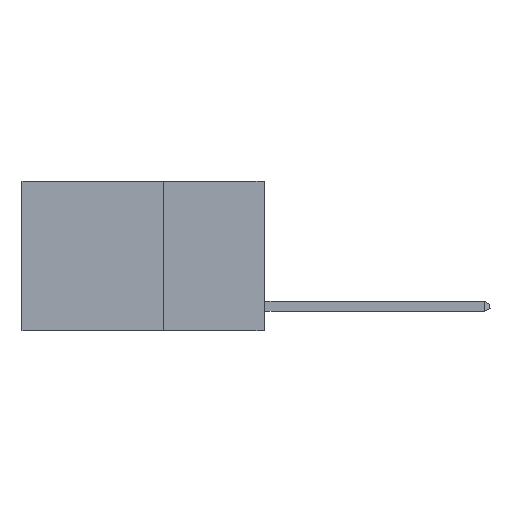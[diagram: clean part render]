
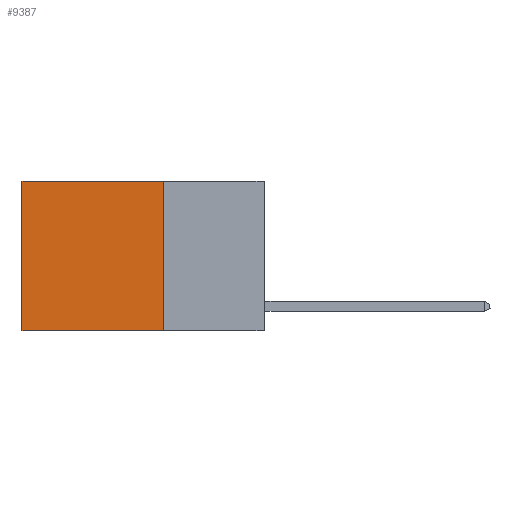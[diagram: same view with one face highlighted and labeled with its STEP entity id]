
A CAD part, left-side view. The second image highlights one B-rep face of the part: STEP entity #9387.
In plain terms, the highlighted planar face has unit normal (-1, 0, 0).
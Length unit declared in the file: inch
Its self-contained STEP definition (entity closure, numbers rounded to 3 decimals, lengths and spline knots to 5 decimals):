
#393 = EDGE_CURVE ( 'NONE', #11661, #764, #10028, .T. ) ;
#699 = EDGE_LOOP ( 'NONE', ( #8748, #8536, #5588, #6928 ) ) ;
#764 = VERTEX_POINT ( 'NONE', #2091 ) ;
#2091 = CARTESIAN_POINT ( 'NONE',  ( 0.2625, 0.6, -0.37 ) ) ;
#2301 = FACE_OUTER_BOUND ( 'NONE', #699, .T. ) ;
#2621 = CARTESIAN_POINT ( 'NONE',  ( 0.2625, 0.25, -0.37 ) ) ;
#3111 = VECTOR ( 'NONE', #11618, 39.37008 ) ;
#3209 = VECTOR ( 'NONE', #6446, 39.37008 ) ;
#3554 = VERTEX_POINT ( 'NONE', #9403 ) ;
#3621 = DIRECTION ( 'NONE',  ( 0., 0., -1. ) ) ;
#3931 = LINE ( 'NONE', #13209, #3209 ) ;
#4444 = VECTOR ( 'NONE', #11052, 39.37008 ) ;
#4874 = CARTESIAN_POINT ( 'NONE',  ( 0.2625, 0.25, 0. ) ) ;
#5588 = ORIENTED_EDGE ( 'NONE', *, *, #9069, .F. ) ;
#6446 = DIRECTION ( 'NONE',  ( 0., 0., -1. ) ) ;
#6928 = ORIENTED_EDGE ( 'NONE', *, *, #12800, .T. ) ;
#7049 = VECTOR ( 'NONE', #12629, 39.37008 ) ;
#8536 = ORIENTED_EDGE ( 'NONE', *, *, #9156, .F. ) ;
#8748 = ORIENTED_EDGE ( 'NONE', *, *, #393, .T. ) ;
#8855 = VERTEX_POINT ( 'NONE', #2621 ) ;
#9069 = EDGE_CURVE ( 'NONE', #3554, #8855, #3931, .T. ) ;
#9156 = EDGE_CURVE ( 'NONE', #8855, #764, #13463, .T. ) ;
#9219 = CARTESIAN_POINT ( 'NONE',  ( 0.2625, 0.25, 0. ) ) ;
#9387 = ADVANCED_FACE ( 'NONE', ( #2301 ), #11439, .F. ) ;
#9403 = CARTESIAN_POINT ( 'NONE',  ( 0.2625, 0.25, 0. ) ) ;
#9899 = AXIS2_PLACEMENT_3D ( 'NONE', #9219, #10354, #3621 ) ;
#10028 = LINE ( 'NONE', #11474, #7049 ) ;
#10354 = DIRECTION ( 'NONE',  ( 1., 0., 0. ) ) ;
#10755 = CARTESIAN_POINT ( 'NONE',  ( 0.2625, 0.6, 0. ) ) ;
#11052 = DIRECTION ( 'NONE',  ( 0., 1., 0. ) ) ;
#11400 = LINE ( 'NONE', #4874, #3111 ) ;
#11439 = PLANE ( 'NONE',  #9899 ) ;
#11474 = CARTESIAN_POINT ( 'NONE',  ( 0.2625, 0.6, 0. ) ) ;
#11618 = DIRECTION ( 'NONE',  ( 0., 1., 0. ) ) ;
#11661 = VERTEX_POINT ( 'NONE', #10755 ) ;
#12629 = DIRECTION ( 'NONE',  ( 0., 0., -1. ) ) ;
#12800 = EDGE_CURVE ( 'NONE', #3554, #11661, #11400, .T. ) ;
#13209 = CARTESIAN_POINT ( 'NONE',  ( 0.2625, 0.25, 0. ) ) ;
#13356 = CARTESIAN_POINT ( 'NONE',  ( 0.2625, 0.25, -0.37 ) ) ;
#13463 = LINE ( 'NONE', #13356, #4444 ) ;
